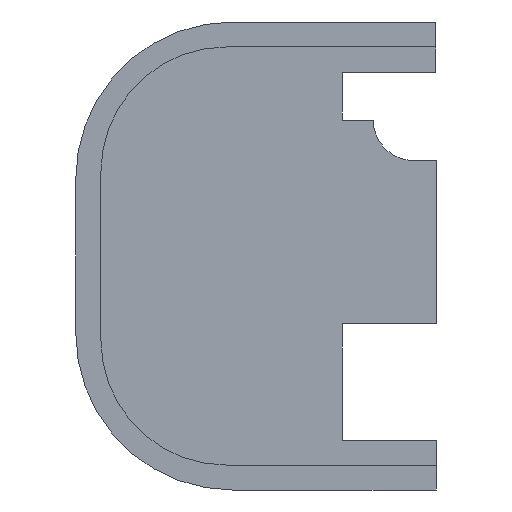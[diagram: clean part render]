
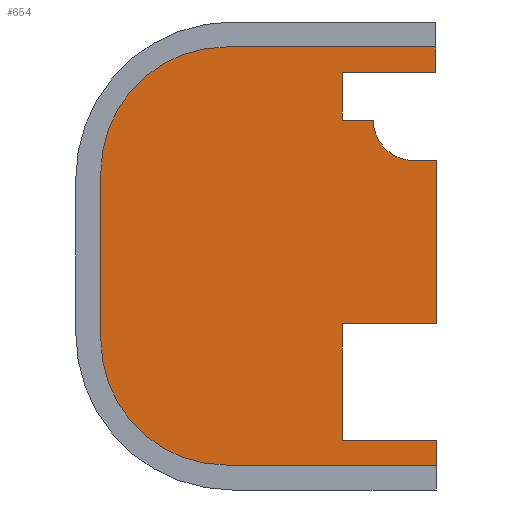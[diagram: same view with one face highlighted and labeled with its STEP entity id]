
A CAD part, left-side view. The second image highlights one B-rep face of the part: STEP entity #654.
In plain terms, the highlighted planar face has unit normal (-1, 0, 0).
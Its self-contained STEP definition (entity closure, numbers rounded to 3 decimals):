
#18=PLANE('',#705);
#45=FACE_OUTER_BOUND('',#80,.T.);
#80=EDGE_LOOP('',(#456,#457,#458,#459,#460,#461,#462,#463,#464,#465,#466,
#467,#468,#469,#470,#471));
#118=LINE('',#949,#197);
#119=LINE('',#951,#198);
#120=LINE('',#953,#199);
#121=LINE('',#955,#200);
#122=LINE('',#957,#201);
#123=LINE('',#959,#202);
#124=LINE('',#961,#203);
#125=LINE('',#965,#204);
#126=LINE('',#967,#205);
#127=LINE('',#969,#206);
#128=LINE('',#971,#207);
#129=LINE('',#973,#208);
#130=LINE('',#977,#209);
#197=VECTOR('',#765,10.);
#198=VECTOR('',#766,10.);
#199=VECTOR('',#767,10.);
#200=VECTOR('',#768,10.);
#201=VECTOR('',#769,10.);
#202=VECTOR('',#770,10.);
#203=VECTOR('',#771,10.);
#204=VECTOR('',#774,10.);
#205=VECTOR('',#775,10.);
#206=VECTOR('',#776,10.);
#207=VECTOR('',#777,10.);
#208=VECTOR('',#778,10.);
#209=VECTOR('',#781,10.);
#277=CIRCLE('',#706,1.647);
#278=CIRCLE('',#707,5.08);
#279=CIRCLE('',#708,5.08);
#294=VERTEX_POINT('',#947);
#295=VERTEX_POINT('',#948);
#296=VERTEX_POINT('',#950);
#297=VERTEX_POINT('',#952);
#298=VERTEX_POINT('',#954);
#299=VERTEX_POINT('',#956);
#300=VERTEX_POINT('',#958);
#301=VERTEX_POINT('',#960);
#302=VERTEX_POINT('',#962);
#303=VERTEX_POINT('',#964);
#304=VERTEX_POINT('',#966);
#305=VERTEX_POINT('',#968);
#306=VERTEX_POINT('',#970);
#307=VERTEX_POINT('',#972);
#308=VERTEX_POINT('',#974);
#309=VERTEX_POINT('',#976);
#359=EDGE_CURVE('',#294,#295,#118,.T.);
#360=EDGE_CURVE('',#296,#294,#119,.T.);
#361=EDGE_CURVE('',#297,#296,#120,.T.);
#362=EDGE_CURVE('',#298,#297,#121,.T.);
#363=EDGE_CURVE('',#299,#298,#122,.T.);
#364=EDGE_CURVE('',#300,#299,#123,.T.);
#365=EDGE_CURVE('',#301,#300,#124,.T.);
#366=EDGE_CURVE('',#302,#301,#277,.T.);
#367=EDGE_CURVE('',#303,#302,#125,.T.);
#368=EDGE_CURVE('',#304,#303,#126,.T.);
#369=EDGE_CURVE('',#305,#304,#127,.T.);
#370=EDGE_CURVE('',#306,#305,#128,.T.);
#371=EDGE_CURVE('',#307,#306,#129,.T.);
#372=EDGE_CURVE('',#308,#307,#278,.T.);
#373=EDGE_CURVE('',#309,#308,#130,.T.);
#374=EDGE_CURVE('',#295,#309,#279,.T.);
#456=ORIENTED_EDGE('',*,*,#359,.F.);
#457=ORIENTED_EDGE('',*,*,#360,.F.);
#458=ORIENTED_EDGE('',*,*,#361,.F.);
#459=ORIENTED_EDGE('',*,*,#362,.F.);
#460=ORIENTED_EDGE('',*,*,#363,.F.);
#461=ORIENTED_EDGE('',*,*,#364,.F.);
#462=ORIENTED_EDGE('',*,*,#365,.F.);
#463=ORIENTED_EDGE('',*,*,#366,.F.);
#464=ORIENTED_EDGE('',*,*,#367,.F.);
#465=ORIENTED_EDGE('',*,*,#368,.F.);
#466=ORIENTED_EDGE('',*,*,#369,.F.);
#467=ORIENTED_EDGE('',*,*,#370,.F.);
#468=ORIENTED_EDGE('',*,*,#371,.F.);
#469=ORIENTED_EDGE('',*,*,#372,.F.);
#470=ORIENTED_EDGE('',*,*,#373,.F.);
#471=ORIENTED_EDGE('',*,*,#374,.F.);
#654=ADVANCED_FACE('',(#45),#18,.T.);
#705=AXIS2_PLACEMENT_3D('',#946,#763,#764);
#706=AXIS2_PLACEMENT_3D('',#963,#772,#773);
#707=AXIS2_PLACEMENT_3D('',#975,#779,#780);
#708=AXIS2_PLACEMENT_3D('',#978,#782,#783);
#763=DIRECTION('center_axis',(-1.,0.,0.));
#764=DIRECTION('ref_axis',(0.,0.,1.));
#765=DIRECTION('',(0.,1.,0.));
#766=DIRECTION('',(0.,0.,-1.));
#767=DIRECTION('',(0.,-1.,0.));
#768=DIRECTION('',(0.,0.,-1.));
#769=DIRECTION('',(0.,1.,0.));
#770=DIRECTION('',(0.,0.,-1.));
#771=DIRECTION('',(0.,-1.,0.));
#772=DIRECTION('center_axis',(-1.,0.,0.));
#773=DIRECTION('ref_axis',(0.,0.,-1.));
#774=DIRECTION('',(0.,-1.,0.));
#775=DIRECTION('',(0.,0.,-1.));
#776=DIRECTION('',(0.,1.,0.));
#777=DIRECTION('',(0.,0.,-1.));
#778=DIRECTION('',(0.,-1.,0.));
#779=DIRECTION('center_axis',(1.,0.,0.));
#780=DIRECTION('ref_axis',(0.,0.,1.));
#781=DIRECTION('',(0.,0.,1.));
#782=DIRECTION('center_axis',(1.,0.,0.));
#783=DIRECTION('ref_axis',(0.,0.,1.));
#946=CARTESIAN_POINT('Origin',(214.305,1.844,18.171));
#947=CARTESIAN_POINT('',(214.305,-5.459,9.701));
#948=CARTESIAN_POINT('',(214.305,3.05,9.701));
#949=CARTESIAN_POINT('',(214.305,-1.807,9.701));
#950=CARTESIAN_POINT('',(214.305,-5.459,10.697));
#951=CARTESIAN_POINT('',(214.305,-5.459,13.431));
#952=CARTESIAN_POINT('',(214.305,-1.65,10.697));
#953=CARTESIAN_POINT('',(214.305,-1.807,10.697));
#954=CARTESIAN_POINT('',(214.305,-1.65,15.421));
#955=CARTESIAN_POINT('',(214.305,-1.65,14.434));
#956=CARTESIAN_POINT('',(214.305,-5.459,15.421));
#957=CARTESIAN_POINT('',(214.305,-1.807,15.421));
#958=CARTESIAN_POINT('',(214.305,-5.459,22.039));
#959=CARTESIAN_POINT('',(214.305,-5.459,18.451));
#960=CARTESIAN_POINT('',(214.305,-4.56,22.039));
#961=CARTESIAN_POINT('',(214.305,-1.807,22.039));
#962=CARTESIAN_POINT('',(214.305,-2.907,23.68));
#963=CARTESIAN_POINT('Origin',(214.305,-4.554,23.686));
#964=CARTESIAN_POINT('',(214.305,-1.65,23.68));
#965=CARTESIAN_POINT('',(214.305,-0.532,23.68));
#966=CARTESIAN_POINT('',(214.305,-1.65,25.595));
#967=CARTESIAN_POINT('',(214.305,-1.65,20.926));
#968=CARTESIAN_POINT('',(214.305,-5.447,25.595));
#969=CARTESIAN_POINT('',(214.305,-1.802,25.595));
#970=CARTESIAN_POINT('',(214.305,-5.447,26.642));
#971=CARTESIAN_POINT('',(214.305,-5.447,22.398));
#972=CARTESIAN_POINT('',(214.305,3.05,26.642));
#973=CARTESIAN_POINT('',(214.305,-1.802,26.642));
#974=CARTESIAN_POINT('',(214.305,8.13,21.562));
#975=CARTESIAN_POINT('Origin',(214.305,3.05,21.562));
#976=CARTESIAN_POINT('',(214.305,8.13,14.781));
#977=CARTESIAN_POINT('',(214.305,8.13,16.476));
#978=CARTESIAN_POINT('Origin',(214.305,3.05,14.781));
